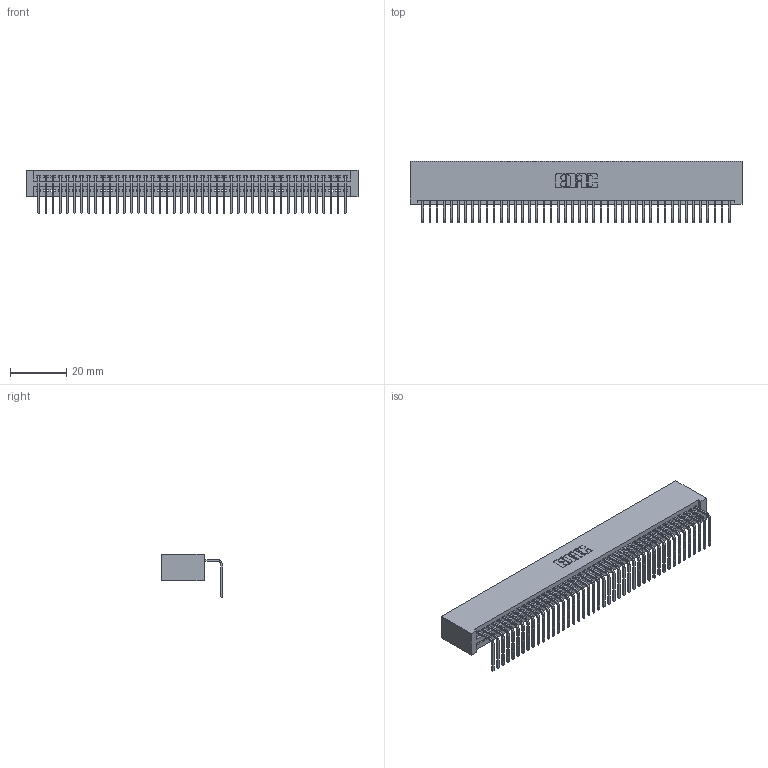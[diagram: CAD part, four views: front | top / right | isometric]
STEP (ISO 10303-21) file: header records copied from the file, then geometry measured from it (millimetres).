
FILE_DESCRIPTION (( 'STEP AP203' ), '1' );
FILE_NAME ('345-044-558-101.STEP', '2019-10-10T16:49:37', ( '' ), ( '' ), 'SwSTEP 2.0', 'SolidWorks 2016', '' );
FILE_SCHEMA (( 'CONFIG_CONTROL_DESIGN' ));
Length unit declared in the file: inch
Products named in the file (3): 345 Part_No Mounting Lugs; 345-292-001_558 Tail - 2; 345-044-558-101
Assembly tree (45 placements, depth 2):
  345-044-558-101
    345 Part_No Mounting Lugs
    345-292-001_558 Tail - 2  x44
Bounding box: 118.36 x 21.83 x 15.37 mm (x, y, z)
Volume: 11989.7 mm3; surface area: 17011.9 mm2
Topology: 45 solids, 45 shells, 2758 faces, 8325 edges, 5490 vertices
Faces by surface type: plane 1924, cylinder 834
Entity records: 32653 total; most frequent: CARTESIAN_POINT 5664, ORIENTED_EDGE 5642, DIRECTION 4937, EDGE_CURVE 2821, LINE 2521, VECTOR 2521, VERTEX_POINT 1878, AXIS2_PLACEMENT_3D 1208
